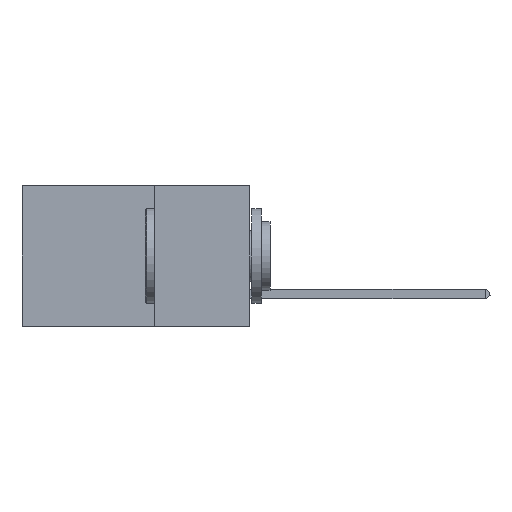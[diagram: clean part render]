
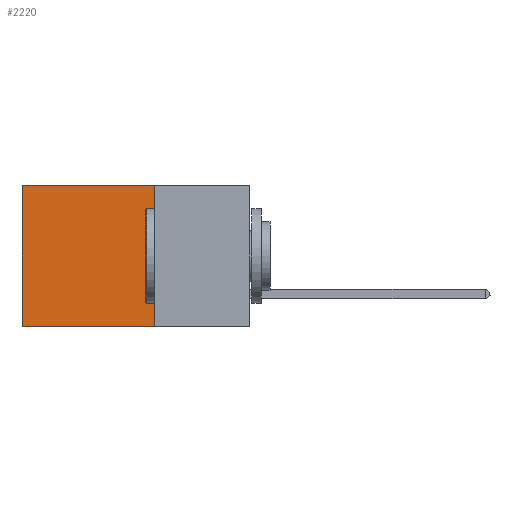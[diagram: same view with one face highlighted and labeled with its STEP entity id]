
A CAD part, left-side view. The second image highlights one B-rep face of the part: STEP entity #2220.
In plain terms, the highlighted planar face has unit normal (-1, 0, 0).
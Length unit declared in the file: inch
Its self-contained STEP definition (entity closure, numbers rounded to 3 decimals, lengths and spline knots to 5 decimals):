
#1060 = DIRECTION ( 'NONE',  ( 1., 0., 0. ) ) ;
#2063 = LINE ( 'NONE', #15339, #15157 ) ;
#2220 = ADVANCED_FACE ( 'NONE', ( #5018 ), #4559, .F. ) ;
#2427 = VERTEX_POINT ( 'NONE', #9026 ) ;
#4559 = PLANE ( 'NONE',  #11207 ) ;
#5018 = FACE_OUTER_BOUND ( 'NONE', #16360, .T. ) ;
#5623 = VECTOR ( 'NONE', #13969, 39.37008 ) ;
#6628 = EDGE_CURVE ( 'NONE', #10766, #2427, #15924, .T. ) ;
#7596 = DIRECTION ( 'NONE',  ( 0., 1., 0. ) ) ;
#8288 = VERTEX_POINT ( 'NONE', #16202 ) ;
#8391 = CARTESIAN_POINT ( 'NONE',  ( 0.2875, 0.6, 0. ) ) ;
#9026 = CARTESIAN_POINT ( 'NONE',  ( 0.2875, 0.6, 0. ) ) ;
#9411 = VERTEX_POINT ( 'NONE', #18336 ) ;
#10229 = ORIENTED_EDGE ( 'NONE', *, *, #6628, .T. ) ;
#10349 = LINE ( 'NONE', #8391, #16946 ) ;
#10766 = VERTEX_POINT ( 'NONE', #18561 ) ;
#11207 = AXIS2_PLACEMENT_3D ( 'NONE', #15318, #1060, #13481 ) ;
#11497 = DIRECTION ( 'NONE',  ( 0., 0., -1. ) ) ;
#13054 = CARTESIAN_POINT ( 'NONE',  ( 0.2875, 0.25, 0. ) ) ;
#13481 = DIRECTION ( 'NONE',  ( 0., 0., -1. ) ) ;
#13969 = DIRECTION ( 'NONE',  ( 0., 1., 0. ) ) ;
#14475 = EDGE_CURVE ( 'NONE', #2427, #8288, #10349, .T. ) ;
#15021 = LINE ( 'NONE', #23044, #5623 ) ;
#15157 = VECTOR ( 'NONE', #11497, 39.37008 ) ;
#15318 = CARTESIAN_POINT ( 'NONE',  ( 0.2875, 0.25, 0. ) ) ;
#15339 = CARTESIAN_POINT ( 'NONE',  ( 0.2875, 0.25, 0. ) ) ;
#15775 = DIRECTION ( 'NONE',  ( 0., 0., -1. ) ) ;
#15924 = LINE ( 'NONE', #13054, #17071 ) ;
#15994 = EDGE_CURVE ( 'NONE', #10766, #9411, #2063, .T. ) ;
#16202 = CARTESIAN_POINT ( 'NONE',  ( 0.2875, 0.6, -0.37 ) ) ;
#16360 = EDGE_LOOP ( 'NONE', ( #16737, #22807, #22715, #10229 ) ) ;
#16737 = ORIENTED_EDGE ( 'NONE', *, *, #14475, .T. ) ;
#16946 = VECTOR ( 'NONE', #15775, 39.37008 ) ;
#17071 = VECTOR ( 'NONE', #7596, 39.37008 ) ;
#18336 = CARTESIAN_POINT ( 'NONE',  ( 0.2875, 0.25, -0.37 ) ) ;
#18561 = CARTESIAN_POINT ( 'NONE',  ( 0.2875, 0.25, 0. ) ) ;
#22259 = EDGE_CURVE ( 'NONE', #9411, #8288, #15021, .T. ) ;
#22715 = ORIENTED_EDGE ( 'NONE', *, *, #15994, .F. ) ;
#22807 = ORIENTED_EDGE ( 'NONE', *, *, #22259, .F. ) ;
#23044 = CARTESIAN_POINT ( 'NONE',  ( 0.2875, 0.25, -0.37 ) ) ;
